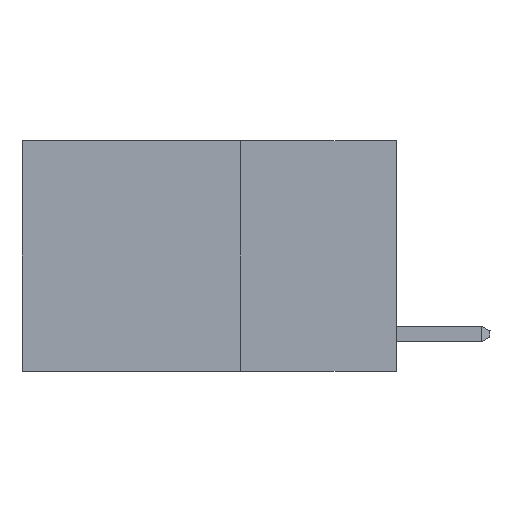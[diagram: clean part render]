
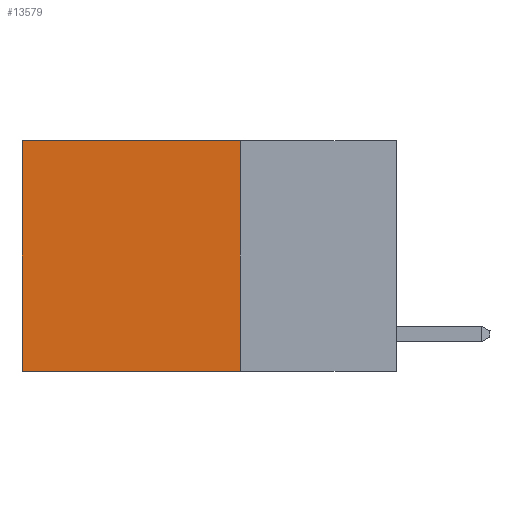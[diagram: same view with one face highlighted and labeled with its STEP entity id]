
A CAD part, left-side view. The second image highlights one B-rep face of the part: STEP entity #13579.
In plain terms, the highlighted planar face has unit normal (-1, 0, 0).
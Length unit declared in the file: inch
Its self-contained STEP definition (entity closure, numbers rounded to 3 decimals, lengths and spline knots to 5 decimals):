
#240 = LINE ( 'NONE', #7104, #1848 ) ;
#405 = LINE ( 'NONE', #7935, #5405 ) ;
#777 = DIRECTION ( 'NONE',  ( 0., 1., 0. ) ) ;
#800 = LINE ( 'NONE', #1853, #6538 ) ;
#808 = ORIENTED_EDGE ( 'NONE', *, *, #6712, .T. ) ;
#924 = DIRECTION ( 'NONE',  ( 0., 0., -1. ) ) ;
#1848 = VECTOR ( 'NONE', #8329, 39.37008 ) ;
#1853 = CARTESIAN_POINT ( 'NONE',  ( 0.2625, 0.25, -0.37 ) ) ;
#1891 = CARTESIAN_POINT ( 'NONE',  ( 0.2625, 0.25, 0. ) ) ;
#2415 = PLANE ( 'NONE',  #8950 ) ;
#2642 = VERTEX_POINT ( 'NONE', #8765 ) ;
#2942 = LINE ( 'NONE', #1891, #10379 ) ;
#3083 = DIRECTION ( 'NONE',  ( 0., 1., 0. ) ) ;
#3797 = CARTESIAN_POINT ( 'NONE',  ( 0.2625, 0.25, -0.37 ) ) ;
#4039 = FACE_OUTER_BOUND ( 'NONE', #13086, .T. ) ;
#5405 = VECTOR ( 'NONE', #924, 39.37008 ) ;
#5868 = DIRECTION ( 'NONE',  ( 0., 0., -1. ) ) ;
#5920 = CARTESIAN_POINT ( 'NONE',  ( 0.2625, 0.25, 0. ) ) ;
#6254 = CARTESIAN_POINT ( 'NONE',  ( 0.2625, 0.25, 0. ) ) ;
#6360 = VERTEX_POINT ( 'NONE', #3797 ) ;
#6362 = EDGE_CURVE ( 'NONE', #14331, #6360, #240, .T. ) ;
#6538 = VECTOR ( 'NONE', #3083, 39.37008 ) ;
#6712 = EDGE_CURVE ( 'NONE', #2642, #9519, #405, .T. ) ;
#6832 = ORIENTED_EDGE ( 'NONE', *, *, #14397, .T. ) ;
#6911 = ORIENTED_EDGE ( 'NONE', *, *, #6362, .F. ) ;
#7104 = CARTESIAN_POINT ( 'NONE',  ( 0.2625, 0.25, 0. ) ) ;
#7935 = CARTESIAN_POINT ( 'NONE',  ( 0.2625, 0.6, 0. ) ) ;
#8329 = DIRECTION ( 'NONE',  ( 0., 0., -1. ) ) ;
#8765 = CARTESIAN_POINT ( 'NONE',  ( 0.2625, 0.6, 0. ) ) ;
#8950 = AXIS2_PLACEMENT_3D ( 'NONE', #5920, #12776, #5868 ) ;
#9519 = VERTEX_POINT ( 'NONE', #11250 ) ;
#10379 = VECTOR ( 'NONE', #777, 39.37008 ) ;
#10635 = EDGE_CURVE ( 'NONE', #6360, #9519, #800, .T. ) ;
#11250 = CARTESIAN_POINT ( 'NONE',  ( 0.2625, 0.6, -0.37 ) ) ;
#12776 = DIRECTION ( 'NONE',  ( 1., 0., 0. ) ) ;
#13086 = EDGE_LOOP ( 'NONE', ( #808, #14795, #6911, #6832 ) ) ;
#13579 = ADVANCED_FACE ( 'NONE', ( #4039 ), #2415, .F. ) ;
#14331 = VERTEX_POINT ( 'NONE', #6254 ) ;
#14397 = EDGE_CURVE ( 'NONE', #14331, #2642, #2942, .T. ) ;
#14795 = ORIENTED_EDGE ( 'NONE', *, *, #10635, .F. ) ;
